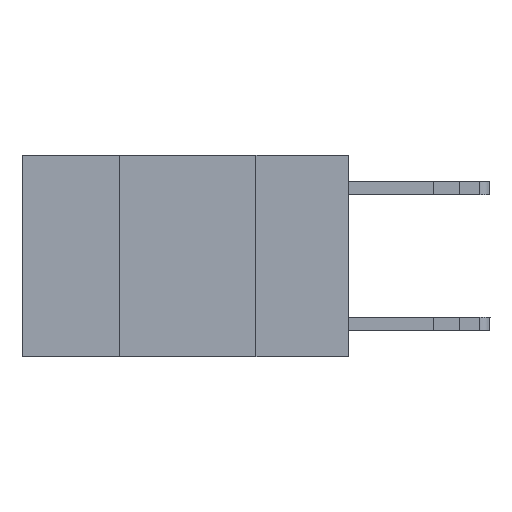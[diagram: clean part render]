
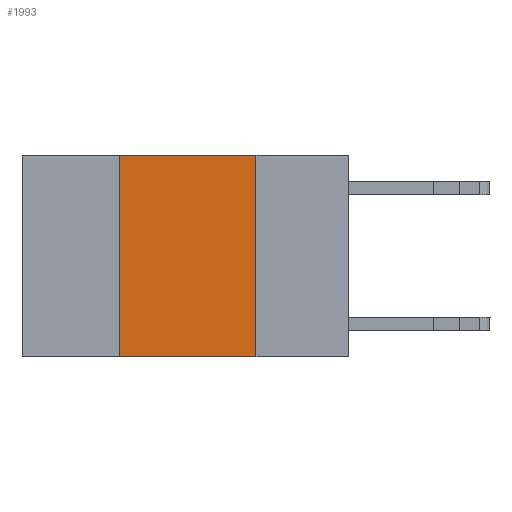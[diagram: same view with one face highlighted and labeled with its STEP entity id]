
A CAD part, left-side view. The second image highlights one B-rep face of the part: STEP entity #1993.
In plain terms, the highlighted planar face has unit normal (-1, 0, 0).
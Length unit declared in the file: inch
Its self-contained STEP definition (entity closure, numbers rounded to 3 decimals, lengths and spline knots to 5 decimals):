
#1363 = EDGE_LOOP ( 'NONE', ( #8879, #4165, #9895, #11636 ) ) ;
#1371 = DIRECTION ( 'NONE',  ( 1., 0., 0. ) ) ;
#1756 = CARTESIAN_POINT ( 'NONE',  ( 0., 0.42, -0.37 ) ) ;
#1971 = VECTOR ( 'NONE', #8453, 39.37008 ) ;
#1993 = ADVANCED_FACE ( 'NONE', ( #3601 ), #5064, .F. ) ;
#3139 = DIRECTION ( 'NONE',  ( 0., -1., 0. ) ) ;
#3299 = VERTEX_POINT ( 'NONE', #1756 ) ;
#3601 = FACE_OUTER_BOUND ( 'NONE', #1363, .T. ) ;
#3754 = CARTESIAN_POINT ( 'NONE',  ( 0., 0.17, 0. ) ) ;
#4096 = LINE ( 'NONE', #10402, #10718 ) ;
#4165 = ORIENTED_EDGE ( 'NONE', *, *, #8969, .F. ) ;
#4193 = CARTESIAN_POINT ( 'NONE',  ( 0., 0.6, 0. ) ) ;
#4346 = CARTESIAN_POINT ( 'NONE',  ( 0., 0.42, 0. ) ) ;
#4360 = LINE ( 'NONE', #7540, #1971 ) ;
#4479 = LINE ( 'NONE', #6872, #9117 ) ;
#5064 = PLANE ( 'NONE',  #7534 ) ;
#5164 = DIRECTION ( 'NONE',  ( 0., 0., -1. ) ) ;
#5191 = VECTOR ( 'NONE', #3139, 39.37008 ) ;
#5253 = DIRECTION ( 'NONE',  ( 0., -1., 0. ) ) ;
#5847 = VERTEX_POINT ( 'NONE', #4346 ) ;
#5923 = DIRECTION ( 'NONE',  ( 0., 0., -1. ) ) ;
#6573 = CARTESIAN_POINT ( 'NONE',  ( 0., 0.6, -0.37 ) ) ;
#6872 = CARTESIAN_POINT ( 'NONE',  ( 0., 0.17, 0. ) ) ;
#7458 = LINE ( 'NONE', #6573, #5191 ) ;
#7534 = AXIS2_PLACEMENT_3D ( 'NONE', #4193, #1371, #5923 ) ;
#7540 = CARTESIAN_POINT ( 'NONE',  ( 0., 0.42, 0. ) ) ;
#7975 = EDGE_CURVE ( 'NONE', #3299, #10128, #7458, .T. ) ;
#8095 = EDGE_CURVE ( 'NONE', #3299, #5847, #4360, .T. ) ;
#8453 = DIRECTION ( 'NONE',  ( 0., 0., 1. ) ) ;
#8594 = VERTEX_POINT ( 'NONE', #3754 ) ;
#8879 = ORIENTED_EDGE ( 'NONE', *, *, #9727, .F. ) ;
#8969 = EDGE_CURVE ( 'NONE', #5847, #8594, #4096, .T. ) ;
#9117 = VECTOR ( 'NONE', #5164, 39.37008 ) ;
#9727 = EDGE_CURVE ( 'NONE', #8594, #10128, #4479, .T. ) ;
#9895 = ORIENTED_EDGE ( 'NONE', *, *, #8095, .F. ) ;
#10128 = VERTEX_POINT ( 'NONE', #11615 ) ;
#10402 = CARTESIAN_POINT ( 'NONE',  ( 0., 0.6, 0. ) ) ;
#10718 = VECTOR ( 'NONE', #5253, 39.37008 ) ;
#11615 = CARTESIAN_POINT ( 'NONE',  ( 0., 0.17, -0.37 ) ) ;
#11636 = ORIENTED_EDGE ( 'NONE', *, *, #7975, .T. ) ;
